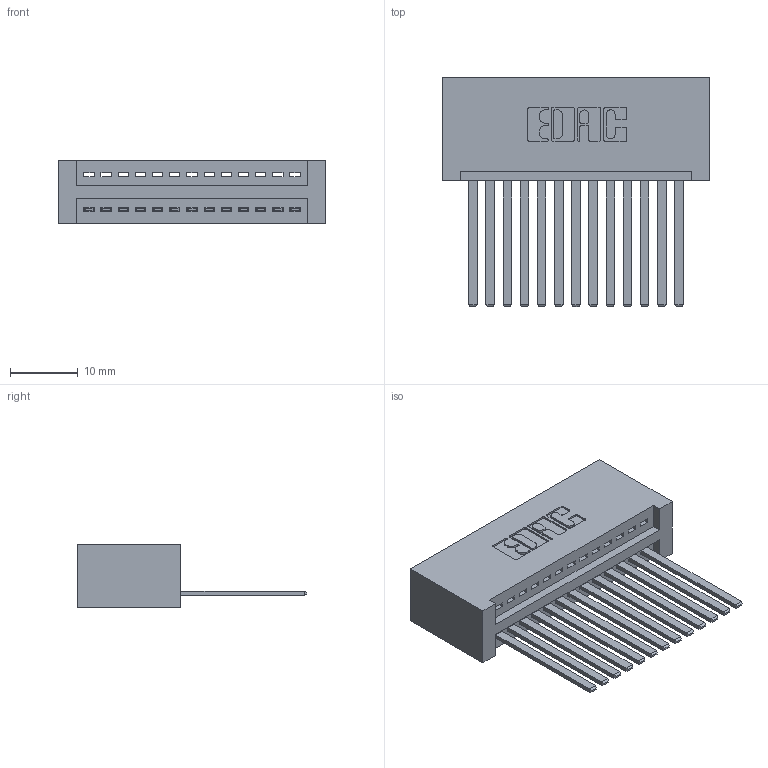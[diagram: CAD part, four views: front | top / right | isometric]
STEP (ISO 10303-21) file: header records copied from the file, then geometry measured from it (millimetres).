
FILE_DESCRIPTION (( 'STEP AP203' ), '1' );
FILE_NAME ('345-013-544-101.STEP', '2019-10-04T04:27:49', ( '' ), ( '' ), 'SwSTEP 2.0', 'SolidWorks 2016', '' );
FILE_SCHEMA (( 'CONFIG_CONTROL_DESIGN' ));
Length unit declared in the file: inch
Products named in the file (3): 345 Part_No Mounting Lugs; 345-013-544-101; 345-292-001_345-293-144
Assembly tree (14 placements, depth 2):
  345-013-544-101
    345 Part_No Mounting Lugs
    345-292-001_345-293-144  x13
Bounding box: 39.62 x 33.96 x 9.4 mm (x, y, z)
Volume: 4260.9 mm3; surface area: 5910.3 mm2
Topology: 14 solids, 14 shells, 794 faces, 2371 edges, 1562 vertices
Faces by surface type: plane 544, cylinder 250
Entity records: 13227 total; most frequent: CARTESIAN_POINT 2299, ORIENTED_EDGE 2246, DIRECTION 2041, EDGE_CURVE 1123, VECTOR 951, LINE 951, VERTEX_POINT 746, AXIS2_PLACEMENT_3D 545
